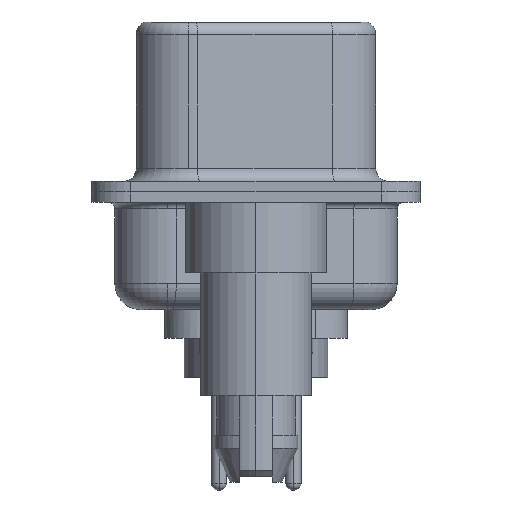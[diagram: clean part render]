
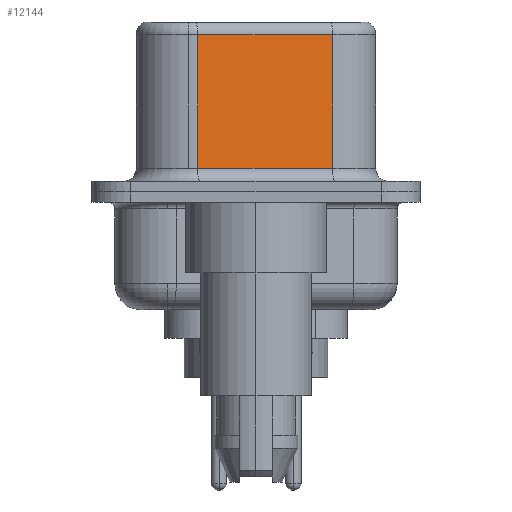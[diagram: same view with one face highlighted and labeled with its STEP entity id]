
A CAD part, left-side view. The second image highlights one B-rep face of the part: STEP entity #12144.
In plain terms, the highlighted planar face has unit normal (-0.985, -0.174, 0).
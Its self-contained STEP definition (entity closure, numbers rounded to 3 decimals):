
#87 = VECTOR ( 'NONE', #7247, 1000. ) ;
#195 = DIRECTION ( 'NONE',  ( -0.174, 0.985, 0. ) ) ;
#1026 = VECTOR ( 'NONE', #5686, 1000. ) ;
#1107 = CARTESIAN_POINT ( 'NONE',  ( 3.67, 2.233, 6.52 ) ) ;
#1338 = CARTESIAN_POINT ( 'NONE',  ( 3.67, 2.233, 6.02 ) ) ;
#2080 = FACE_OUTER_BOUND ( 'NONE', #3051, .T. ) ;
#2085 = CARTESIAN_POINT ( 'NONE',  ( 4.58, -2.927, 6.02 ) ) ;
#2187 = DIRECTION ( 'NONE',  ( -0.174, 0.985, 0. ) ) ;
#2442 = VERTEX_POINT ( 'NONE', #12322 ) ;
#2475 = DIRECTION ( 'NONE',  ( 0., 0., -1. ) ) ;
#2499 = LINE ( 'NONE', #2085, #14362 ) ;
#3051 = EDGE_LOOP ( 'NONE', ( #8899, #9959, #13372, #9311 ) ) ;
#3229 = LINE ( 'NONE', #12886, #87 ) ;
#3283 = AXIS2_PLACEMENT_3D ( 'NONE', #10634, #7242, #195 ) ;
#4125 = LINE ( 'NONE', #10835, #1026 ) ;
#4339 = VERTEX_POINT ( 'NONE', #9811 ) ;
#5686 = DIRECTION ( 'NONE',  ( 0.174, -0.985, 0. ) ) ;
#6347 = EDGE_CURVE ( 'NONE', #7854, #2442, #11029, .T. ) ;
#6780 = EDGE_CURVE ( 'NONE', #11000, #4339, #3229, .T. ) ;
#7242 = DIRECTION ( 'NONE',  ( 0.985, 0.174, 0. ) ) ;
#7247 = DIRECTION ( 'NONE',  ( 0., 0., -1. ) ) ;
#7570 = EDGE_CURVE ( 'NONE', #2442, #4339, #4125, .T. ) ;
#7854 = VERTEX_POINT ( 'NONE', #1338 ) ;
#8030 = VECTOR ( 'NONE', #2475, 1000. ) ;
#8359 = EDGE_CURVE ( 'NONE', #11000, #7854, #2499, .T. ) ;
#8899 = ORIENTED_EDGE ( 'NONE', *, *, #6780, .F. ) ;
#9311 = ORIENTED_EDGE ( 'NONE', *, *, #7570, .T. ) ;
#9811 = CARTESIAN_POINT ( 'NONE',  ( 4.58, -2.927, 0.9 ) ) ;
#9959 = ORIENTED_EDGE ( 'NONE', *, *, #8359, .T. ) ;
#10634 = CARTESIAN_POINT ( 'NONE',  ( 4.58, -2.927, 6.52 ) ) ;
#10835 = CARTESIAN_POINT ( 'NONE',  ( 4.58, -2.927, 0.9 ) ) ;
#11000 = VERTEX_POINT ( 'NONE', #12914 ) ;
#11029 = LINE ( 'NONE', #1107, #8030 ) ;
#12144 = ADVANCED_FACE ( 'NONE', ( #2080 ), #13968, .F. ) ;
#12322 = CARTESIAN_POINT ( 'NONE',  ( 3.67, 2.233, 0.9 ) ) ;
#12886 = CARTESIAN_POINT ( 'NONE',  ( 4.58, -2.927, 6.52 ) ) ;
#12914 = CARTESIAN_POINT ( 'NONE',  ( 4.58, -2.927, 6.02 ) ) ;
#13372 = ORIENTED_EDGE ( 'NONE', *, *, #6347, .T. ) ;
#13968 = PLANE ( 'NONE',  #3283 ) ;
#14362 = VECTOR ( 'NONE', #2187, 1000. ) ;
